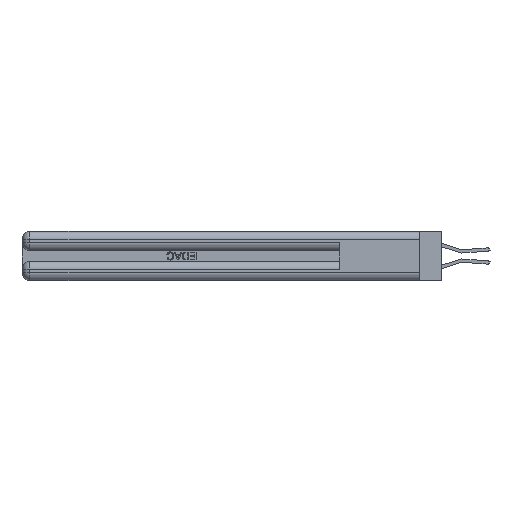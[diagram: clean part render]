
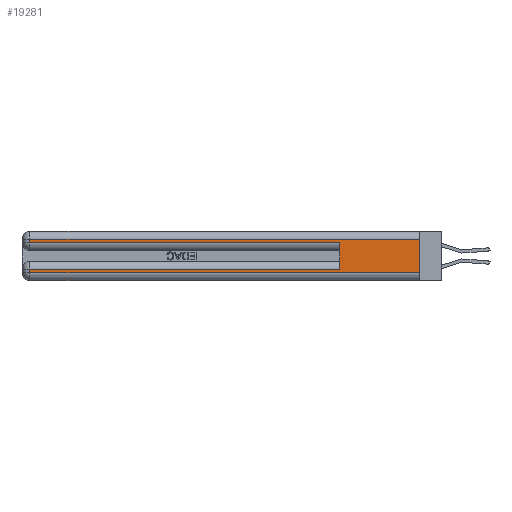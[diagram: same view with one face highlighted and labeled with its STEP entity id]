
A CAD part, left-side view. The second image highlights one B-rep face of the part: STEP entity #19281.
In plain terms, the highlighted planar face has unit normal (-1, 0, 0).
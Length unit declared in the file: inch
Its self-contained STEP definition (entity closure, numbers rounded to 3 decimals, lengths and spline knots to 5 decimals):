
#615 = EDGE_CURVE ( 'NONE', #4838, #46384, #41494, .T. ) ;
#3114 = EDGE_CURVE ( 'NONE', #46241, #28688, #5440, .T. ) ;
#4071 = DIRECTION ( 'NONE',  ( 0., 0., -1. ) ) ;
#4838 = VERTEX_POINT ( 'NONE', #19800 ) ;
#5440 = LINE ( 'NONE', #33473, #19168 ) ;
#5779 = CARTESIAN_POINT ( 'NONE',  ( 0., 0., 0.06 ) ) ;
#6388 = LINE ( 'NONE', #39494, #39209 ) ;
#6410 = CARTESIAN_POINT ( 'NONE',  ( 0., 2.94, 0.085 ) ) ;
#7241 = DIRECTION ( 'NONE',  ( 1., 0., 0. ) ) ;
#7579 = CARTESIAN_POINT ( 'NONE',  ( 0., 0.6, 0.145 ) ) ;
#9082 = CARTESIAN_POINT ( 'NONE',  ( 0., 0., 0.085 ) ) ;
#10181 = LINE ( 'NONE', #7579, #13216 ) ;
#13216 = VECTOR ( 'NONE', #44612, 39.37008 ) ;
#14928 = CARTESIAN_POINT ( 'NONE',  ( 0., 0., 0.37 ) ) ;
#17977 = CARTESIAN_POINT ( 'NONE',  ( 0., 0., 0.31 ) ) ;
#18940 = PLANE ( 'NONE',  #48721 ) ;
#19168 = VECTOR ( 'NONE', #22115, 39.37008 ) ;
#19281 = ADVANCED_FACE ( 'NONE', ( #19494 ), #18940, .F. ) ;
#19494 = FACE_OUTER_BOUND ( 'NONE', #20310, .T. ) ;
#19800 = CARTESIAN_POINT ( 'NONE',  ( 0., 2.94, 0.285 ) ) ;
#20310 = EDGE_LOOP ( 'NONE', ( #26761, #24713, #35626, #33431, #24658, #25088, #27693, #32409 ) ) ;
#21008 = CARTESIAN_POINT ( 'NONE',  ( 0., 2.94, 0.31 ) ) ;
#21873 = LINE ( 'NONE', #49122, #43305 ) ;
#22115 = DIRECTION ( 'NONE',  ( 0., 0., -1. ) ) ;
#23058 = CARTESIAN_POINT ( 'NONE',  ( 0., 0., 0.37 ) ) ;
#23329 = EDGE_CURVE ( 'NONE', #29912, #31596, #6388, .T. ) ;
#23722 = CARTESIAN_POINT ( 'NONE',  ( 0., 2.94, 0.37 ) ) ;
#24360 = CARTESIAN_POINT ( 'NONE',  ( 0., 0.6, 0.085 ) ) ;
#24437 = DIRECTION ( 'NONE',  ( 0., 1., 0. ) ) ;
#24613 = VECTOR ( 'NONE', #4071, 39.37008 ) ;
#24658 = ORIENTED_EDGE ( 'NONE', *, *, #43190, .F. ) ;
#24713 = ORIENTED_EDGE ( 'NONE', *, *, #23329, .T. ) ;
#25088 = ORIENTED_EDGE ( 'NONE', *, *, #39897, .T. ) ;
#26547 = DIRECTION ( 'NONE',  ( 0., -1., 0. ) ) ;
#26761 = ORIENTED_EDGE ( 'NONE', *, *, #30716, .F. ) ;
#27563 = DIRECTION ( 'NONE',  ( 0., 0., -1. ) ) ;
#27693 = ORIENTED_EDGE ( 'NONE', *, *, #3114, .T. ) ;
#28688 = VERTEX_POINT ( 'NONE', #36118 ) ;
#29912 = VERTEX_POINT ( 'NONE', #17977 ) ;
#30716 = EDGE_CURVE ( 'NONE', #29912, #37923, #37737, .T. ) ;
#30874 = EDGE_CURVE ( 'NONE', #31596, #4838, #33570, .T. ) ;
#31596 = VERTEX_POINT ( 'NONE', #21008 ) ;
#32395 = VECTOR ( 'NONE', #27563, 39.37008 ) ;
#32409 = ORIENTED_EDGE ( 'NONE', *, *, #46491, .T. ) ;
#33431 = ORIENTED_EDGE ( 'NONE', *, *, #615, .T. ) ;
#33473 = CARTESIAN_POINT ( 'NONE',  ( 0., 2.94, 0.37 ) ) ;
#33570 = LINE ( 'NONE', #23722, #32395 ) ;
#34851 = DIRECTION ( 'NONE',  ( 0., 1., 0. ) ) ;
#35626 = ORIENTED_EDGE ( 'NONE', *, *, #30874, .T. ) ;
#36118 = CARTESIAN_POINT ( 'NONE',  ( 0., 2.94, 0.06 ) ) ;
#37027 = VECTOR ( 'NONE', #24437, 39.37008 ) ;
#37126 = VERTEX_POINT ( 'NONE', #24360 ) ;
#37737 = LINE ( 'NONE', #23058, #24613 ) ;
#37923 = VERTEX_POINT ( 'NONE', #5779 ) ;
#39209 = VECTOR ( 'NONE', #34851, 39.37008 ) ;
#39494 = CARTESIAN_POINT ( 'NONE',  ( 0., 0., 0.31 ) ) ;
#39897 = EDGE_CURVE ( 'NONE', #37126, #46241, #39963, .T. ) ;
#39963 = LINE ( 'NONE', #9082, #37027 ) ;
#40106 = CARTESIAN_POINT ( 'NONE',  ( 0., 0.6, 0.285 ) ) ;
#41232 = DIRECTION ( 'NONE',  ( 0., -1., 0. ) ) ;
#41494 = LINE ( 'NONE', #41869, #46895 ) ;
#41869 = CARTESIAN_POINT ( 'NONE',  ( 0., 0., 0.285 ) ) ;
#43190 = EDGE_CURVE ( 'NONE', #37126, #46384, #10181, .T. ) ;
#43305 = VECTOR ( 'NONE', #41232, 39.37008 ) ;
#44612 = DIRECTION ( 'NONE',  ( 0., 0., 1. ) ) ;
#45797 = DIRECTION ( 'NONE',  ( 0., 0., -1. ) ) ;
#46241 = VERTEX_POINT ( 'NONE', #6410 ) ;
#46384 = VERTEX_POINT ( 'NONE', #40106 ) ;
#46491 = EDGE_CURVE ( 'NONE', #28688, #37923, #21873, .T. ) ;
#46895 = VECTOR ( 'NONE', #26547, 39.37008 ) ;
#48721 = AXIS2_PLACEMENT_3D ( 'NONE', #14928, #7241, #45797 ) ;
#49122 = CARTESIAN_POINT ( 'NONE',  ( 0., 0., 0.06 ) ) ;
